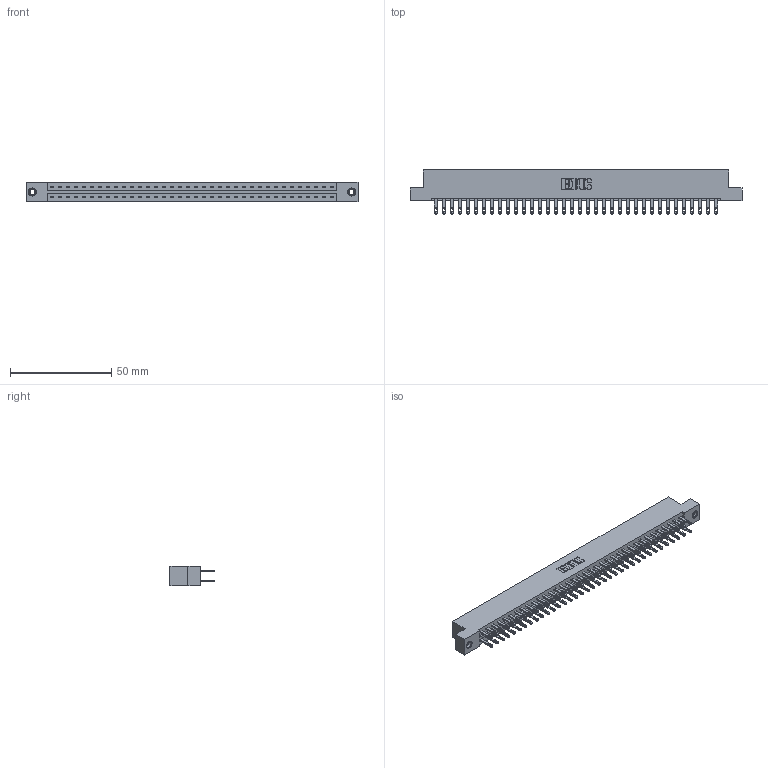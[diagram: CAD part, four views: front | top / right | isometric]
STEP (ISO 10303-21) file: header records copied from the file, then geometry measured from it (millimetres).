
FILE_DESCRIPTION (( 'STEP AP203' ), '1' );
FILE_NAME ('833-072-500-207.STEP', '2020-06-05T13:31:54', ( '' ), ( '' ), 'SwSTEP 2.0', 'SolidWorks 2020', '' );
FILE_SCHEMA (( 'CONFIG_CONTROL_DESIGN' ));
Length unit declared in the file: inch
Products named in the file (4): 345-292-001_345-293-100; 833-072-500-207; 345-250-001_345-250-005-103; 833 Part_Flush - .156 Dia - TI
Assembly tree (75 placements, depth 2):
  833-072-500-207
    833 Part_Flush - .156 Dia - TI
    345-292-001_345-293-100  x72
    345-250-001_345-250-005-103  x2
Bounding box: 164.19 x 21.85 x 9.4 mm (x, y, z)
Volume: 16912.8 mm3; surface area: 20757.1 mm2
Topology: 75 solids, 75 shells, 3630 faces, 11031 edges, 7346 vertices
Faces by surface type: plane 2262, cylinder 1352, cone 12, torus 4
Entity records: 25052 total; most frequent: CARTESIAN_POINT 4141, ORIENTED_EDGE 4070, DIRECTION 3581, EDGE_CURVE 2035, LINE 1883, VECTOR 1883, VERTEX_POINT 1352, AXIS2_PLACEMENT_3D 849
